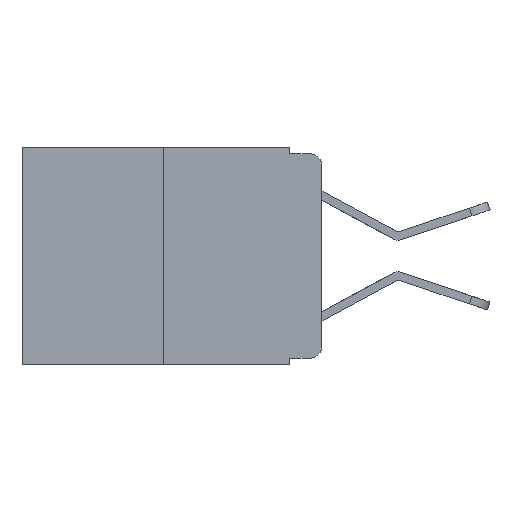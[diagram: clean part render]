
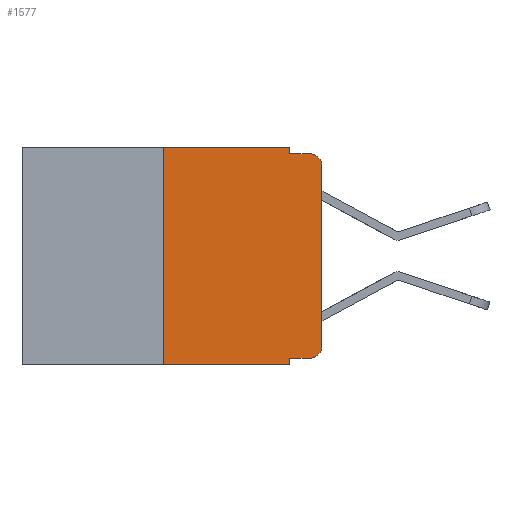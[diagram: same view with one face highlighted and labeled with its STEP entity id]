
A CAD part, left-side view. The second image highlights one B-rep face of the part: STEP entity #1577.
In plain terms, the highlighted planar face has unit normal (-1, 0, 0).
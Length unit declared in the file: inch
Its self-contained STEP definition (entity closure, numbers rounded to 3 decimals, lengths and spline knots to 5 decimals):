
#489 = LINE ( 'NONE', #4461, #9571 ) ;
#502 = LINE ( 'NONE', #11070, #2457 ) ;
#693 = CARTESIAN_POINT ( 'NONE',  ( 0., 0.051, -0.343 ) ) ;
#884 = VERTEX_POINT ( 'NONE', #1358 ) ;
#1005 = CARTESIAN_POINT ( 'NONE',  ( 0., 0.02, -0.03 ) ) ;
#1182 = DIRECTION ( 'NONE',  ( 0., 0., -1. ) ) ;
#1358 = CARTESIAN_POINT ( 'NONE',  ( 0., 0.051, -0.01 ) ) ;
#1421 = DIRECTION ( 'NONE',  ( 0., 0., -1. ) ) ;
#1487 = ORIENTED_EDGE ( 'NONE', *, *, #11013, .T. ) ;
#1577 = ADVANCED_FACE ( 'NONE', ( #6494 ), #10767, .F. ) ;
#1705 = AXIS2_PLACEMENT_3D ( 'NONE', #11682, #9593, #9513 ) ;
#1952 = DIRECTION ( 'NONE',  ( 0., -1., 0. ) ) ;
#2024 = DIRECTION ( 'NONE',  ( 0., -1., 0. ) ) ;
#2201 = ORIENTED_EDGE ( 'NONE', *, *, #3993, .T. ) ;
#2212 = VERTEX_POINT ( 'NONE', #9104 ) ;
#2218 = CARTESIAN_POINT ( 'NONE',  ( 0., 0.473, 0. ) ) ;
#2395 = VECTOR ( 'NONE', #2661, 39.37008 ) ;
#2457 = VECTOR ( 'NONE', #1421, 39.37008 ) ;
#2521 = LINE ( 'NONE', #10152, #2395 ) ;
#2661 = DIRECTION ( 'NONE',  ( 0., 0., 1. ) ) ;
#3093 = CARTESIAN_POINT ( 'NONE',  ( 0., 0.25, 0. ) ) ;
#3222 = LINE ( 'NONE', #11548, #11143 ) ;
#3337 = CARTESIAN_POINT ( 'NONE',  ( 0., 0.25, -0.343 ) ) ;
#3340 = CIRCLE ( 'NONE', #11595, 0.02 ) ;
#3798 = ORIENTED_EDGE ( 'NONE', *, *, #11996, .F. ) ;
#3976 = EDGE_CURVE ( 'NONE', #13613, #12102, #8347, .T. ) ;
#3993 = EDGE_CURVE ( 'NONE', #9669, #13668, #8403, .T. ) ;
#4025 = CARTESIAN_POINT ( 'NONE',  ( 0., 0.051, 0. ) ) ;
#4230 = ORIENTED_EDGE ( 'NONE', *, *, #3976, .F. ) ;
#4390 = EDGE_CURVE ( 'NONE', #9870, #5937, #489, .T. ) ;
#4461 = CARTESIAN_POINT ( 'NONE',  ( 0., 0.051, -0.333 ) ) ;
#4732 = VERTEX_POINT ( 'NONE', #12619 ) ;
#5060 = EDGE_LOOP ( 'NONE', ( #7968, #7147, #3798, #11841, #4230, #11779, #2201, #9077, #7042, #1487 ) ) ;
#5876 = VECTOR ( 'NONE', #2024, 39.37008 ) ;
#5937 = VERTEX_POINT ( 'NONE', #10699 ) ;
#6200 = VECTOR ( 'NONE', #6520, 39.37008 ) ;
#6494 = FACE_OUTER_BOUND ( 'NONE', #5060, .T. ) ;
#6520 = DIRECTION ( 'NONE',  ( 0., -1., 0. ) ) ;
#6577 = DIRECTION ( 'NONE',  ( 0., -1., 0. ) ) ;
#6752 = CARTESIAN_POINT ( 'NONE',  ( 0., 0., -0.03 ) ) ;
#6897 = CARTESIAN_POINT ( 'NONE',  ( 0., 0.051, -0.333 ) ) ;
#7042 = ORIENTED_EDGE ( 'NONE', *, *, #4390, .T. ) ;
#7147 = ORIENTED_EDGE ( 'NONE', *, *, #8155, .T. ) ;
#7200 = EDGE_CURVE ( 'NONE', #9669, #13613, #3222, .T. ) ;
#7578 = LINE ( 'NONE', #11839, #6200 ) ;
#7968 = ORIENTED_EDGE ( 'NONE', *, *, #12033, .T. ) ;
#8155 = EDGE_CURVE ( 'NONE', #13267, #4732, #3340, .T. ) ;
#8347 = LINE ( 'NONE', #10505, #5876 ) ;
#8403 = LINE ( 'NONE', #12627, #12999 ) ;
#8855 = CIRCLE ( 'NONE', #1705, 0.02 ) ;
#9025 = EDGE_CURVE ( 'NONE', #12102, #884, #502, .T. ) ;
#9077 = ORIENTED_EDGE ( 'NONE', *, *, #9651, .F. ) ;
#9104 = CARTESIAN_POINT ( 'NONE',  ( 0., 0., -0.313 ) ) ;
#9513 = DIRECTION ( 'NONE',  ( 0., 0., -1. ) ) ;
#9571 = VECTOR ( 'NONE', #6577, 39.37008 ) ;
#9593 = DIRECTION ( 'NONE',  ( -1., 0., 0. ) ) ;
#9651 = EDGE_CURVE ( 'NONE', #9870, #13668, #10404, .T. ) ;
#9669 = VERTEX_POINT ( 'NONE', #3337 ) ;
#9845 = AXIS2_PLACEMENT_3D ( 'NONE', #2218, #11807, #1182 ) ;
#9870 = VERTEX_POINT ( 'NONE', #6897 ) ;
#9887 = CARTESIAN_POINT ( 'NONE',  ( 0., 0.051, 0. ) ) ;
#10152 = CARTESIAN_POINT ( 'NONE',  ( 0., 0., 0. ) ) ;
#10404 = LINE ( 'NONE', #4025, #10525 ) ;
#10435 = DIRECTION ( 'NONE',  ( 0., 0., 1. ) ) ;
#10505 = CARTESIAN_POINT ( 'NONE',  ( 0., 0.473, 0. ) ) ;
#10525 = VECTOR ( 'NONE', #12551, 39.37008 ) ;
#10699 = CARTESIAN_POINT ( 'NONE',  ( 0., 0.02, -0.333 ) ) ;
#10767 = PLANE ( 'NONE',  #9845 ) ;
#11013 = EDGE_CURVE ( 'NONE', #5937, #2212, #8855, .T. ) ;
#11070 = CARTESIAN_POINT ( 'NONE',  ( 0., 0.051, 0. ) ) ;
#11143 = VECTOR ( 'NONE', #10435, 39.37008 ) ;
#11548 = CARTESIAN_POINT ( 'NONE',  ( 0., 0.25, 0. ) ) ;
#11595 = AXIS2_PLACEMENT_3D ( 'NONE', #1005, #11714, #11777 ) ;
#11682 = CARTESIAN_POINT ( 'NONE',  ( 0., 0.02, -0.313 ) ) ;
#11714 = DIRECTION ( 'NONE',  ( -1., 0., 0. ) ) ;
#11777 = DIRECTION ( 'NONE',  ( 0., 0., -1. ) ) ;
#11779 = ORIENTED_EDGE ( 'NONE', *, *, #7200, .F. ) ;
#11807 = DIRECTION ( 'NONE',  ( 1., 0., 0. ) ) ;
#11839 = CARTESIAN_POINT ( 'NONE',  ( 0., 0.051, -0.01 ) ) ;
#11841 = ORIENTED_EDGE ( 'NONE', *, *, #9025, .F. ) ;
#11996 = EDGE_CURVE ( 'NONE', #884, #4732, #7578, .T. ) ;
#12033 = EDGE_CURVE ( 'NONE', #2212, #13267, #2521, .T. ) ;
#12102 = VERTEX_POINT ( 'NONE', #9887 ) ;
#12551 = DIRECTION ( 'NONE',  ( 0., 0., -1. ) ) ;
#12619 = CARTESIAN_POINT ( 'NONE',  ( 0., 0.02, -0.01 ) ) ;
#12627 = CARTESIAN_POINT ( 'NONE',  ( 0., 0.473, -0.343 ) ) ;
#12999 = VECTOR ( 'NONE', #1952, 39.37008 ) ;
#13267 = VERTEX_POINT ( 'NONE', #6752 ) ;
#13613 = VERTEX_POINT ( 'NONE', #3093 ) ;
#13668 = VERTEX_POINT ( 'NONE', #693 ) ;
